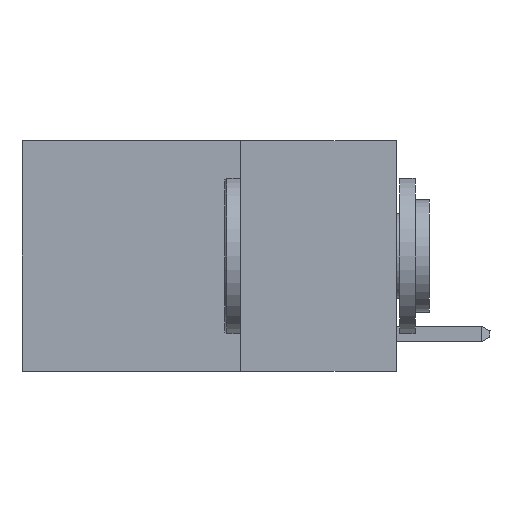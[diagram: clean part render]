
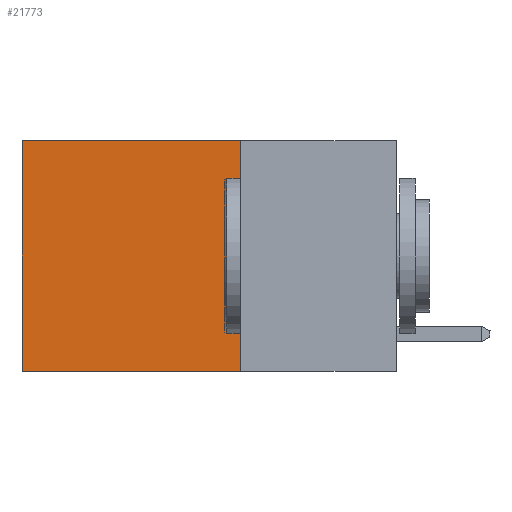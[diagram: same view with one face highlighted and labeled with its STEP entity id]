
A CAD part, left-side view. The second image highlights one B-rep face of the part: STEP entity #21773.
In plain terms, the highlighted planar face has unit normal (-1, 0, 0).
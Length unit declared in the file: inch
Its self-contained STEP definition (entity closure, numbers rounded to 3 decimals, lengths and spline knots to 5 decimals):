
#470 = VECTOR ( 'NONE', #10267, 39.37008 ) ;
#725 = CARTESIAN_POINT ( 'NONE',  ( 0.2625, 0.25, 0. ) ) ;
#2217 = VERTEX_POINT ( 'NONE', #9929 ) ;
#2793 = EDGE_CURVE ( 'NONE', #9656, #9682, #16143, .T. ) ;
#4013 = CARTESIAN_POINT ( 'NONE',  ( 0.2625, 0.25, 0. ) ) ;
#4970 = DIRECTION ( 'NONE',  ( 1., 0., 0. ) ) ;
#5292 = VECTOR ( 'NONE', #9637, 39.37008 ) ;
#5363 = CARTESIAN_POINT ( 'NONE',  ( 0.2625, 0.6, -0.37 ) ) ;
#5962 = LINE ( 'NONE', #4013, #470 ) ;
#6021 = CARTESIAN_POINT ( 'NONE',  ( 0.2625, 0.6, 0. ) ) ;
#6829 = ORIENTED_EDGE ( 'NONE', *, *, #15523, .T. ) ;
#7622 = EDGE_CURVE ( 'NONE', #25161, #9682, #19079, .T. ) ;
#7790 = LINE ( 'NONE', #18070, #23258 ) ;
#9637 = DIRECTION ( 'NONE',  ( 0., 1., 0. ) ) ;
#9651 = VECTOR ( 'NONE', #22232, 39.37008 ) ;
#9656 = VERTEX_POINT ( 'NONE', #16466 ) ;
#9682 = VERTEX_POINT ( 'NONE', #5363 ) ;
#9929 = CARTESIAN_POINT ( 'NONE',  ( 0.2625, 0.25, 0. ) ) ;
#9938 = EDGE_CURVE ( 'NONE', #2217, #9656, #5962, .T. ) ;
#10267 = DIRECTION ( 'NONE',  ( 0., 0., -1. ) ) ;
#11667 = ORIENTED_EDGE ( 'NONE', *, *, #2793, .F. ) ;
#12141 = DIRECTION ( 'NONE',  ( 0., 1., 0. ) ) ;
#12250 = ORIENTED_EDGE ( 'NONE', *, *, #7622, .T. ) ;
#12410 = CARTESIAN_POINT ( 'NONE',  ( 0.2625, 0.6, 0. ) ) ;
#14083 = AXIS2_PLACEMENT_3D ( 'NONE', #725, #4970, #19194 ) ;
#15438 = FACE_OUTER_BOUND ( 'NONE', #18572, .T. ) ;
#15523 = EDGE_CURVE ( 'NONE', #2217, #25161, #7790, .T. ) ;
#16143 = LINE ( 'NONE', #21690, #5292 ) ;
#16466 = CARTESIAN_POINT ( 'NONE',  ( 0.2625, 0.25, -0.37 ) ) ;
#17181 = PLANE ( 'NONE',  #14083 ) ;
#18070 = CARTESIAN_POINT ( 'NONE',  ( 0.2625, 0.25, 0. ) ) ;
#18572 = EDGE_LOOP ( 'NONE', ( #12250, #11667, #25134, #6829 ) ) ;
#19079 = LINE ( 'NONE', #6021, #9651 ) ;
#19194 = DIRECTION ( 'NONE',  ( 0., 0., -1. ) ) ;
#21690 = CARTESIAN_POINT ( 'NONE',  ( 0.2625, 0.25, -0.37 ) ) ;
#21773 = ADVANCED_FACE ( 'NONE', ( #15438 ), #17181, .F. ) ;
#22232 = DIRECTION ( 'NONE',  ( 0., 0., -1. ) ) ;
#23258 = VECTOR ( 'NONE', #12141, 39.37008 ) ;
#25134 = ORIENTED_EDGE ( 'NONE', *, *, #9938, .F. ) ;
#25161 = VERTEX_POINT ( 'NONE', #12410 ) ;
